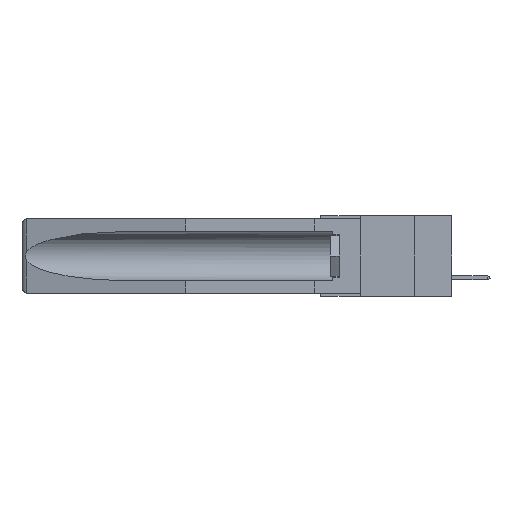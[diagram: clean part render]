
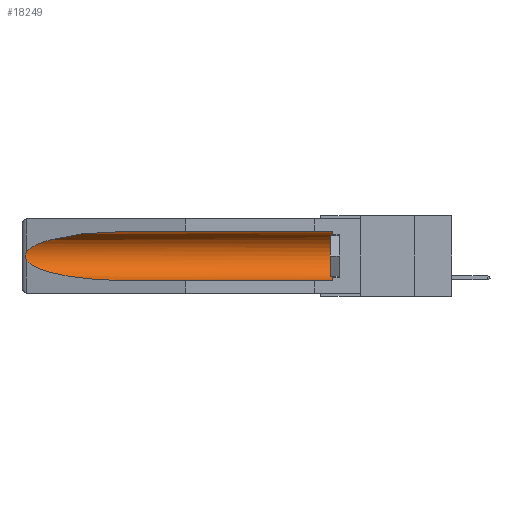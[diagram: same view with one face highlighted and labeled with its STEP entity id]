
A CAD part, left-side view. The second image highlights one B-rep face of the part: STEP entity #18249.
In plain terms, the highlighted cylindrical face has radius 2.857 mm (diameter 5.715 mm), a partial arc.
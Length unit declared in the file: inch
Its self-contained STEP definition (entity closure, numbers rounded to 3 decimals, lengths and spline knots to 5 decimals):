
#19 = VERTEX_POINT ( 'NONE', #9281 ) ;
#298 = LINE ( 'NONE', #2866, #10740 ) ;
#339 = CARTESIAN_POINT ( 'NONE',  ( 0.26537, 1.52718, -0.14972 ) ) ;
#365 = CARTESIAN_POINT ( 'NONE',  ( 0.2675, 1.53308, -0.17534 ) ) ;
#584 = CARTESIAN_POINT ( 'NONE',  ( 0.2675, 1.53308, -0.16763 ) ) ;
#592 = EDGE_CURVE ( 'NONE', #1747, #19, #298, .T. ) ;
#702 = CARTESIAN_POINT ( 'NONE',  ( 0.155, 1.07973, -0.284 ) ) ;
#1444 = FACE_OUTER_BOUND ( 'NONE', #4270, .T. ) ;
#1588 = CARTESIAN_POINT ( 'NONE',  ( 0.155, -0.30754, -0.059 ) ) ;
#1601 = ORIENTED_EDGE ( 'NONE', *, *, #21985, .T. ) ;
#1659 = DIRECTION ( 'NONE',  ( 0., 1., 0. ) ) ;
#1747 = VERTEX_POINT ( 'NONE', #15920 ) ;
#2063 = CARTESIAN_POINT ( 'NONE',  ( 0.25451, 1.48313, -0.09465 ) ) ;
#2300 = CARTESIAN_POINT ( 'NONE',  ( 0.155, 0.126, -0.1715 ) ) ;
#2866 = CARTESIAN_POINT ( 'NONE',  ( 0.155, -0.30754, -0.284 ) ) ;
#3732 = EDGE_CURVE ( 'NONE', #19150, #20410, #19758, .T. ) ;
#3793 = CARTESIAN_POINT ( 'NONE',  ( 0.155, 1.07973, -0.059 ) ) ;
#3839 = VERTEX_POINT ( 'NONE', #13893 ) ;
#4270 = EDGE_LOOP ( 'NONE', ( #15964, #1601, #17841, #13333, #8708, #5523 ) ) ;
#4773 = CARTESIAN_POINT ( 'NONE',  ( 0.155, 0.126, -0.059 ) ) ;
#4934 = VECTOR ( 'NONE', #1659, 39.37008 ) ;
#5275 = CARTESIAN_POINT ( 'NONE',  ( 0.155, -0.30754, -0.1715 ) ) ;
#5523 = ORIENTED_EDGE ( 'NONE', *, *, #3732, .T. ) ;
#5716 = CARTESIAN_POINT ( 'NONE',  ( 0.26654, 1.53092, -0.15636 ) ) ;
#5940 =( BOUNDED_CURVE ( )  B_SPLINE_CURVE ( 3, ( #7216, #21125, #2063, #339 ),
 .UNSPECIFIED., .F., .F. ) 
 B_SPLINE_CURVE_WITH_KNOTS ( ( 4, 4 ),
 ( 4.71239, 6.08839 ),
 .UNSPECIFIED. ) 
 CURVE ( )  GEOMETRIC_REPRESENTATION_ITEM ( )  RATIONAL_B_SPLINE_CURVE ( ( 1., 0.848, 0.848, 1. ) ) 
 REPRESENTATION_ITEM ( '' )  );
#7216 = CARTESIAN_POINT ( 'NONE',  ( 0.155, 1.07973, -0.059 ) ) ;
#7367 = CARTESIAN_POINT ( 'NONE',  ( 0.26537, 1.52718, -0.19328 ) ) ;
#7582 = CARTESIAN_POINT ( 'NONE',  ( 0.25451, 1.48313, -0.24835 ) ) ;
#7951 = DIRECTION ( 'NONE',  ( 0., 1., 0. ) ) ;
#8708 = ORIENTED_EDGE ( 'NONE', *, *, #12232, .T. ) ;
#8986 = CARTESIAN_POINT ( 'NONE',  ( 0.26597, 1.5296, -0.19026 ) ) ;
#9200 = CARTESIAN_POINT ( 'NONE',  ( 0.2673, 1.5327, -0.16383 ) ) ;
#9281 = CARTESIAN_POINT ( 'NONE',  ( 0.155, 1.07973, -0.284 ) ) ;
#10740 = VECTOR ( 'NONE', #7951, 39.37008 ) ;
#11363 = AXIS2_PLACEMENT_3D ( 'NONE', #5275, #12221, #17334 ) ;
#11402 = DIRECTION ( 'NONE',  ( 0., 0., 1. ) ) ;
#11857 = CARTESIAN_POINT ( 'NONE',  ( 0.26537, 1.52718, -0.14972 ) ) ;
#12221 = DIRECTION ( 'NONE',  ( 0., 1., 0. ) ) ;
#12232 = EDGE_CURVE ( 'NONE', #1747, #19150, #21671, .T. ) ;
#12357 = CARTESIAN_POINT ( 'NONE',  ( 0.2673, 1.53269, -0.17917 ) ) ;
#12606 = EDGE_CURVE ( 'NONE', #20410, #13543, #5940, .T. ) ;
#13333 = ORIENTED_EDGE ( 'NONE', *, *, #592, .F. ) ;
#13543 = VERTEX_POINT ( 'NONE', #11857 ) ;
#13893 = CARTESIAN_POINT ( 'NONE',  ( 0.26537, 1.52718, -0.19328 ) ) ;
#14238 = CARTESIAN_POINT ( 'NONE',  ( 0.26537, 1.52718, -0.19328 ) ) ;
#14288 = EDGE_CURVE ( 'NONE', #3839, #19, #19677, .T. ) ;
#14312 = CARTESIAN_POINT ( 'NONE',  ( 0.26655, 1.53094, -0.18657 ) ) ;
#15618 = AXIS2_PLACEMENT_3D ( 'NONE', #2300, #21703, #11402 ) ;
#15890 = CARTESIAN_POINT ( 'NONE',  ( 0.26597, 1.52961, -0.15275 ) ) ;
#15920 = CARTESIAN_POINT ( 'NONE',  ( 0.155, 0.126, -0.284 ) ) ;
#15964 = ORIENTED_EDGE ( 'NONE', *, *, #12606, .T. ) ;
#16009 = CARTESIAN_POINT ( 'NONE',  ( 0.21114, 1.30732, -0.284 ) ) ;
#17310 = CYLINDRICAL_SURFACE ( 'NONE', #11363, 0.1125 ) ;
#17334 = DIRECTION ( 'NONE',  ( 0., 0., 1. ) ) ;
#17835 = CARTESIAN_POINT ( 'NONE',  ( 0.26537, 1.52718, -0.14972 ) ) ;
#17841 = ORIENTED_EDGE ( 'NONE', *, *, #14288, .T. ) ;
#18249 = ADVANCED_FACE ( 'NONE', ( #1444 ), #17310, .F. ) ;
#19150 = VERTEX_POINT ( 'NONE', #4773 ) ;
#19677 =( BOUNDED_CURVE ( )  B_SPLINE_CURVE ( 3, ( #7367, #7582, #16009, #702 ),
 .UNSPECIFIED., .F., .F. ) 
 B_SPLINE_CURVE_WITH_KNOTS ( ( 4, 4 ),
 ( 0.1948, 1.5708 ),
 .UNSPECIFIED. ) 
 CURVE ( )  GEOMETRIC_REPRESENTATION_ITEM ( )  RATIONAL_B_SPLINE_CURVE ( ( 1., 0.848, 0.848, 1. ) ) 
 REPRESENTATION_ITEM ( '' )  );
#19758 = LINE ( 'NONE', #1588, #4934 ) ;
#20403 = B_SPLINE_CURVE_WITH_KNOTS ( 'NONE', 3,
 ( #17835, #15890, #5716, #9200, #584, #365, #12357, #14312, #8986, #14238 ),
 .UNSPECIFIED., .F., .F.,
 ( 4, 2, 2, 2, 4 ),
 ( 0., 0.00029, 0.00058, 0.00087, 0.00117 ),
 .UNSPECIFIED. ) ;
#20410 = VERTEX_POINT ( 'NONE', #3793 ) ;
#21125 = CARTESIAN_POINT ( 'NONE',  ( 0.21114, 1.30732, -0.059 ) ) ;
#21671 = CIRCLE ( 'NONE', #15618, 0.1125 ) ;
#21703 = DIRECTION ( 'NONE',  ( 0., -1., 0. ) ) ;
#21985 = EDGE_CURVE ( 'NONE', #13543, #3839, #20403, .T. ) ;
